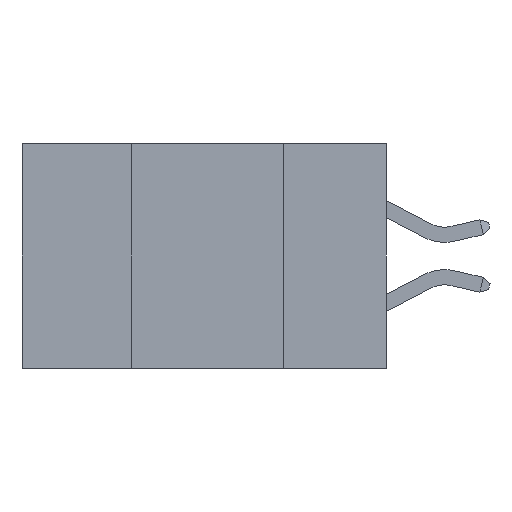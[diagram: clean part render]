
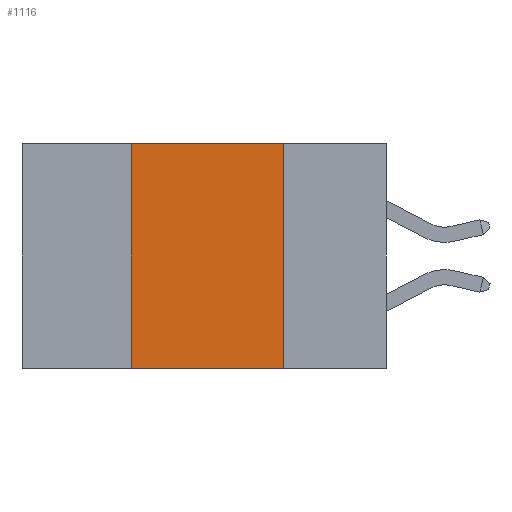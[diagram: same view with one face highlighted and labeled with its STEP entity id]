
A CAD part, left-side view. The second image highlights one B-rep face of the part: STEP entity #1116.
In plain terms, the highlighted planar face has unit normal (-1, 0, 0).
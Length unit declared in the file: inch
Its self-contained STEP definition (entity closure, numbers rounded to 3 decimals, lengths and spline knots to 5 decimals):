
#554 = FACE_OUTER_BOUND ( 'NONE', #8735, .T. ) ;
#889 = VERTEX_POINT ( 'NONE', #2004 ) ;
#1116 = ADVANCED_FACE ( 'NONE', ( #554 ), #9442, .F. ) ;
#1829 = VECTOR ( 'NONE', #8114, 39.37008 ) ;
#1972 = VERTEX_POINT ( 'NONE', #6871 ) ;
#2004 = CARTESIAN_POINT ( 'NONE',  ( 0., 0.17, 0. ) ) ;
#2485 = VECTOR ( 'NONE', #10004, 39.37008 ) ;
#2816 = CARTESIAN_POINT ( 'NONE',  ( 0., 0.17, -0.37 ) ) ;
#3013 = VECTOR ( 'NONE', #5672, 39.37008 ) ;
#3208 = CARTESIAN_POINT ( 'NONE',  ( 0., 0.42, 0. ) ) ;
#5229 = EDGE_CURVE ( 'NONE', #1972, #6463, #8149, .T. ) ;
#5672 = DIRECTION ( 'NONE',  ( 0., 0., -1. ) ) ;
#6103 = CARTESIAN_POINT ( 'NONE',  ( 0., 0.17, -0.37 ) ) ;
#6290 = ORIENTED_EDGE ( 'NONE', *, *, #10382, .F. ) ;
#6386 = CARTESIAN_POINT ( 'NONE',  ( 0., 0.6, -0.37 ) ) ;
#6432 = DIRECTION ( 'NONE',  ( 0., -1., 0. ) ) ;
#6463 = VERTEX_POINT ( 'NONE', #2816 ) ;
#6871 = CARTESIAN_POINT ( 'NONE',  ( 0., 0.42, -0.37 ) ) ;
#7593 = AXIS2_PLACEMENT_3D ( 'NONE', #11244, #9426, #11194 ) ;
#7935 = CARTESIAN_POINT ( 'NONE',  ( 0., 0.42, -0.37 ) ) ;
#8114 = DIRECTION ( 'NONE',  ( 0., 0., 1. ) ) ;
#8149 = LINE ( 'NONE', #6386, #13623 ) ;
#8578 = ORIENTED_EDGE ( 'NONE', *, *, #5229, .T. ) ;
#8735 = EDGE_LOOP ( 'NONE', ( #12330, #9556, #6290, #8578 ) ) ;
#9251 = EDGE_CURVE ( 'NONE', #889, #6463, #11686, .T. ) ;
#9426 = DIRECTION ( 'NONE',  ( 1., 0., 0. ) ) ;
#9442 = PLANE ( 'NONE',  #7593 ) ;
#9497 = CARTESIAN_POINT ( 'NONE',  ( 0., 0.6, 0. ) ) ;
#9498 = EDGE_CURVE ( 'NONE', #9864, #889, #13841, .T. ) ;
#9556 = ORIENTED_EDGE ( 'NONE', *, *, #9498, .F. ) ;
#9864 = VERTEX_POINT ( 'NONE', #3208 ) ;
#10004 = DIRECTION ( 'NONE',  ( 0., -1., 0. ) ) ;
#10382 = EDGE_CURVE ( 'NONE', #1972, #9864, #10574, .T. ) ;
#10574 = LINE ( 'NONE', #7935, #1829 ) ;
#11194 = DIRECTION ( 'NONE',  ( 0., 0., -1. ) ) ;
#11244 = CARTESIAN_POINT ( 'NONE',  ( 0., 0.6, 0. ) ) ;
#11686 = LINE ( 'NONE', #6103, #3013 ) ;
#12330 = ORIENTED_EDGE ( 'NONE', *, *, #9251, .F. ) ;
#13623 = VECTOR ( 'NONE', #6432, 39.37008 ) ;
#13841 = LINE ( 'NONE', #9497, #2485 ) ;
